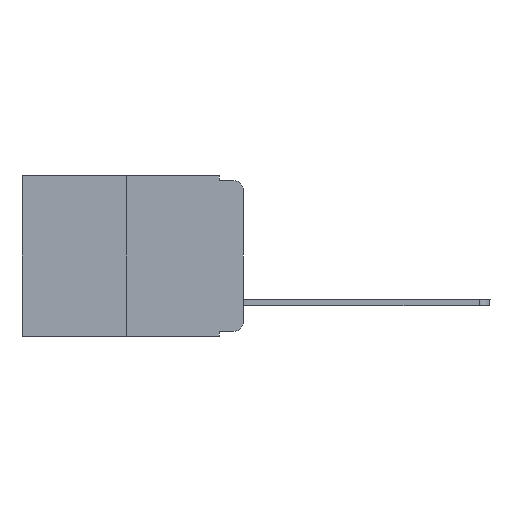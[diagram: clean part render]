
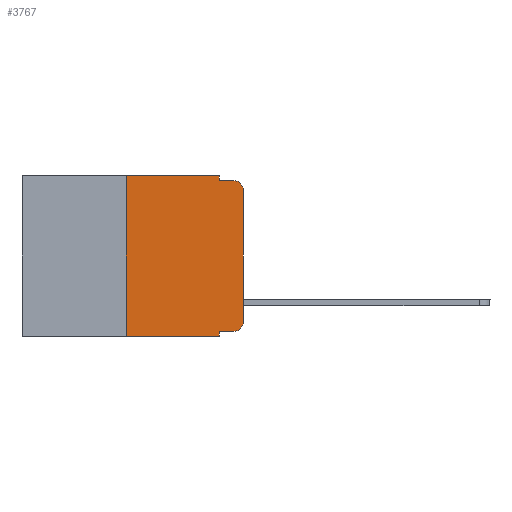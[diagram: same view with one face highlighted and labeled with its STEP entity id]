
A CAD part, left-side view. The second image highlights one B-rep face of the part: STEP entity #3767.
In plain terms, the highlighted planar face has unit normal (-1, 0, 0).
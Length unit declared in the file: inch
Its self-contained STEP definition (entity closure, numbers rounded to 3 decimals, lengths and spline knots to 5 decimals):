
#137 = DIRECTION ( 'NONE',  ( 0., -1., 0. ) ) ;
#303 = DIRECTION ( 'NONE',  ( 0., 0., 1. ) ) ;
#368 = VERTEX_POINT ( 'NONE', #3287 ) ;
#430 = EDGE_CURVE ( 'NONE', #6329, #11947, #9294, .T. ) ;
#460 = CARTESIAN_POINT ( 'NONE',  ( 0., 0.473, -0.343 ) ) ;
#547 = LINE ( 'NONE', #11845, #6397 ) ;
#872 = PLANE ( 'NONE',  #12283 ) ;
#1003 = DIRECTION ( 'NONE',  ( 0., 0., -1. ) ) ;
#1461 = LINE ( 'NONE', #460, #8997 ) ;
#1546 = VECTOR ( 'NONE', #137, 39.37008 ) ;
#1606 = CARTESIAN_POINT ( 'NONE',  ( 0., 0.25, 0. ) ) ;
#1621 = DIRECTION ( 'NONE',  ( -1., 0., 0. ) ) ;
#2090 = DIRECTION ( 'NONE',  ( 0., -1., 0. ) ) ;
#2108 = EDGE_CURVE ( 'NONE', #4157, #7596, #9391, .T. ) ;
#2672 = ORIENTED_EDGE ( 'NONE', *, *, #5191, .F. ) ;
#2693 = DIRECTION ( 'NONE',  ( 0., -1., 0. ) ) ;
#2720 = ORIENTED_EDGE ( 'NONE', *, *, #9473, .T. ) ;
#2826 = CARTESIAN_POINT ( 'NONE',  ( 0., 0.02, -0.01 ) ) ;
#2901 = EDGE_CURVE ( 'NONE', #7205, #368, #5880, .T. ) ;
#2963 = DIRECTION ( 'NONE',  ( 0., 0., -1. ) ) ;
#3287 = CARTESIAN_POINT ( 'NONE',  ( 0., 0.051, -0.01 ) ) ;
#3302 = VECTOR ( 'NONE', #12013, 39.37008 ) ;
#3767 = ADVANCED_FACE ( 'NONE', ( #5969 ), #872, .F. ) ;
#4036 = DIRECTION ( 'NONE',  ( 0., 0., 1. ) ) ;
#4097 = CARTESIAN_POINT ( 'NONE',  ( 0., 0.25, -0.343 ) ) ;
#4157 = VERTEX_POINT ( 'NONE', #10682 ) ;
#4594 = ORIENTED_EDGE ( 'NONE', *, *, #2108, .T. ) ;
#4836 = EDGE_CURVE ( 'NONE', #7596, #9101, #6020, .T. ) ;
#4856 = AXIS2_PLACEMENT_3D ( 'NONE', #10026, #7163, #2963 ) ;
#4870 = CARTESIAN_POINT ( 'NONE',  ( 0., 0.051, 0. ) ) ;
#5037 = ORIENTED_EDGE ( 'NONE', *, *, #4836, .T. ) ;
#5191 = EDGE_CURVE ( 'NONE', #8577, #7205, #9299, .T. ) ;
#5298 = CARTESIAN_POINT ( 'NONE',  ( 0., 0.051, 0. ) ) ;
#5405 = CARTESIAN_POINT ( 'NONE',  ( 0., 0., 0. ) ) ;
#5611 = CIRCLE ( 'NONE', #12421, 0.02 ) ;
#5880 = LINE ( 'NONE', #4870, #3302 ) ;
#5922 = DIRECTION ( 'NONE',  ( 0., 0., -1. ) ) ;
#5969 = FACE_OUTER_BOUND ( 'NONE', #12260, .T. ) ;
#5980 = ORIENTED_EDGE ( 'NONE', *, *, #2901, .F. ) ;
#6020 = LINE ( 'NONE', #5405, #7811 ) ;
#6134 = VECTOR ( 'NONE', #2090, 39.37008 ) ;
#6329 = VERTEX_POINT ( 'NONE', #6717 ) ;
#6397 = VECTOR ( 'NONE', #2693, 39.37008 ) ;
#6675 = ORIENTED_EDGE ( 'NONE', *, *, #12131, .F. ) ;
#6717 = CARTESIAN_POINT ( 'NONE',  ( 0., 0.051, -0.333 ) ) ;
#7112 = CARTESIAN_POINT ( 'NONE',  ( 0., 0.051, -0.01 ) ) ;
#7151 = CARTESIAN_POINT ( 'NONE',  ( 0., 0.473, 0. ) ) ;
#7163 = DIRECTION ( 'NONE',  ( -1., 0., 0. ) ) ;
#7205 = VERTEX_POINT ( 'NONE', #10951 ) ;
#7232 = CARTESIAN_POINT ( 'NONE',  ( 0., 0.473, 0. ) ) ;
#7596 = VERTEX_POINT ( 'NONE', #13002 ) ;
#7811 = VECTOR ( 'NONE', #303, 39.37008 ) ;
#8017 = DIRECTION ( 'NONE',  ( 1., 0., 0. ) ) ;
#8109 = LINE ( 'NONE', #12315, #12403 ) ;
#8128 = ORIENTED_EDGE ( 'NONE', *, *, #430, .F. ) ;
#8206 = VERTEX_POINT ( 'NONE', #4097 ) ;
#8577 = VERTEX_POINT ( 'NONE', #1606 ) ;
#8866 = ORIENTED_EDGE ( 'NONE', *, *, #10797, .F. ) ;
#8997 = VECTOR ( 'NONE', #12563, 39.37008 ) ;
#9101 = VERTEX_POINT ( 'NONE', #12199 ) ;
#9247 = LINE ( 'NONE', #7112, #1546 ) ;
#9294 = LINE ( 'NONE', #5298, #11017 ) ;
#9299 = LINE ( 'NONE', #7232, #6134 ) ;
#9322 = ORIENTED_EDGE ( 'NONE', *, *, #11877, .T. ) ;
#9391 = CIRCLE ( 'NONE', #4856, 0.02 ) ;
#9427 = DIRECTION ( 'NONE',  ( 0., 0., -1. ) ) ;
#9473 = EDGE_CURVE ( 'NONE', #6329, #4157, #547, .T. ) ;
#10026 = CARTESIAN_POINT ( 'NONE',  ( 0., 0.02, -0.313 ) ) ;
#10037 = CARTESIAN_POINT ( 'NONE',  ( 0., 0.051, -0.343 ) ) ;
#10256 = ORIENTED_EDGE ( 'NONE', *, *, #12653, .T. ) ;
#10682 = CARTESIAN_POINT ( 'NONE',  ( 0., 0.02, -0.333 ) ) ;
#10797 = EDGE_CURVE ( 'NONE', #8206, #8577, #8109, .T. ) ;
#10951 = CARTESIAN_POINT ( 'NONE',  ( 0., 0.051, 0. ) ) ;
#11017 = VECTOR ( 'NONE', #9427, 39.37008 ) ;
#11845 = CARTESIAN_POINT ( 'NONE',  ( 0., 0.051, -0.333 ) ) ;
#11877 = EDGE_CURVE ( 'NONE', #9101, #13182, #5611, .T. ) ;
#11947 = VERTEX_POINT ( 'NONE', #10037 ) ;
#12013 = DIRECTION ( 'NONE',  ( 0., 0., -1. ) ) ;
#12131 = EDGE_CURVE ( 'NONE', #368, #13182, #9247, .T. ) ;
#12199 = CARTESIAN_POINT ( 'NONE',  ( 0., 0., -0.03 ) ) ;
#12260 = EDGE_LOOP ( 'NONE', ( #5037, #9322, #6675, #5980, #2672, #8866, #10256, #8128, #2720, #4594 ) ) ;
#12283 = AXIS2_PLACEMENT_3D ( 'NONE', #7151, #8017, #1003 ) ;
#12315 = CARTESIAN_POINT ( 'NONE',  ( 0., 0.25, 0. ) ) ;
#12403 = VECTOR ( 'NONE', #4036, 39.37008 ) ;
#12421 = AXIS2_PLACEMENT_3D ( 'NONE', #13058, #1621, #5922 ) ;
#12563 = DIRECTION ( 'NONE',  ( 0., -1., 0. ) ) ;
#12653 = EDGE_CURVE ( 'NONE', #8206, #11947, #1461, .T. ) ;
#13002 = CARTESIAN_POINT ( 'NONE',  ( 0., 0., -0.313 ) ) ;
#13058 = CARTESIAN_POINT ( 'NONE',  ( 0., 0.02, -0.03 ) ) ;
#13182 = VERTEX_POINT ( 'NONE', #2826 ) ;
